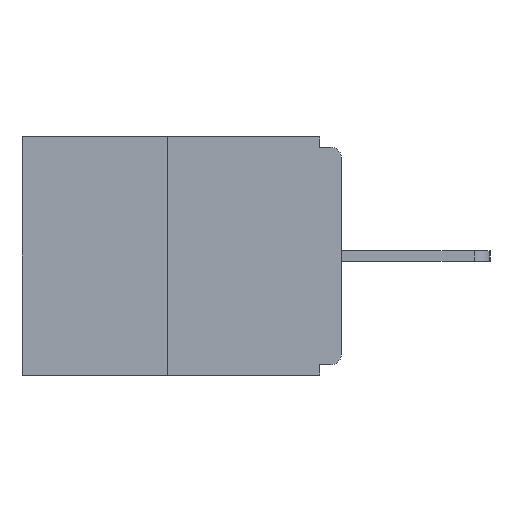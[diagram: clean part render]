
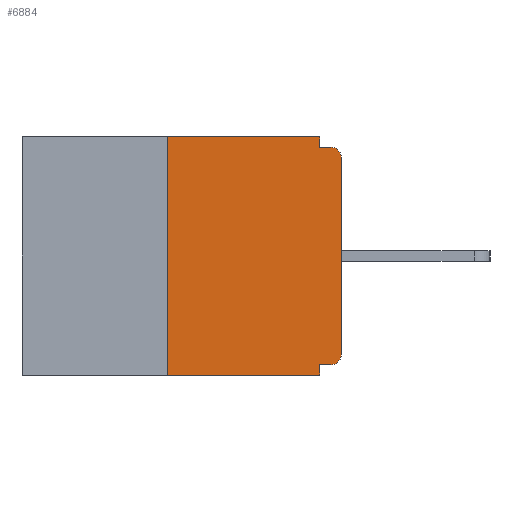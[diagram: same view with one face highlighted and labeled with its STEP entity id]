
A CAD part, left-side view. The second image highlights one B-rep face of the part: STEP entity #6884.
In plain terms, the highlighted planar face has unit normal (-1, 0, 0).
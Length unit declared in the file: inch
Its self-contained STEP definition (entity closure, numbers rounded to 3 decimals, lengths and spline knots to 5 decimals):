
#340 = CARTESIAN_POINT ( 'NONE',  ( 0., 0.031, 0. ) ) ;
#347 = DIRECTION ( 'NONE',  ( 0., 0., 1. ) ) ;
#388 = CARTESIAN_POINT ( 'NONE',  ( 0., 0.031, -0.343 ) ) ;
#733 = CARTESIAN_POINT ( 'NONE',  ( 0., 0.015, -0.313 ) ) ;
#848 = DIRECTION ( 'NONE',  ( 1., 0., 0. ) ) ;
#870 = AXIS2_PLACEMENT_3D ( 'NONE', #733, #18341, #8312 ) ;
#927 = VECTOR ( 'NONE', #15662, 39.37008 ) ;
#994 = CARTESIAN_POINT ( 'NONE',  ( 0., 0.031, 0. ) ) ;
#1183 = EDGE_CURVE ( 'NONE', #24235, #23084, #2751, .T. ) ;
#1205 = EDGE_CURVE ( 'NONE', #11519, #16282, #13908, .T. ) ;
#1241 = LINE ( 'NONE', #2749, #23325 ) ;
#1253 = CARTESIAN_POINT ( 'NONE',  ( 0., 0.031, -0.343 ) ) ;
#1765 = LINE ( 'NONE', #5658, #927 ) ;
#1881 = VERTEX_POINT ( 'NONE', #23646 ) ;
#2054 = LINE ( 'NONE', #388, #7546 ) ;
#2749 = CARTESIAN_POINT ( 'NONE',  ( 0., 0., -0.328 ) ) ;
#2751 = LINE ( 'NONE', #994, #20434 ) ;
#3595 = ORIENTED_EDGE ( 'NONE', *, *, #22627, .T. ) ;
#3606 = ORIENTED_EDGE ( 'NONE', *, *, #17704, .F. ) ;
#4128 = VECTOR ( 'NONE', #10276, 39.37008 ) ;
#4635 = LINE ( 'NONE', #17953, #11554 ) ;
#5385 = DIRECTION ( 'NONE',  ( 0., -1., 0. ) ) ;
#5658 = CARTESIAN_POINT ( 'NONE',  ( 0., 0., 0. ) ) ;
#5837 = ORIENTED_EDGE ( 'NONE', *, *, #10570, .F. ) ;
#6764 = AXIS2_PLACEMENT_3D ( 'NONE', #18196, #848, #8554 ) ;
#6884 = ADVANCED_FACE ( 'NONE', ( #14138 ), #20104, .F. ) ;
#7546 = VECTOR ( 'NONE', #21428, 39.37008 ) ;
#7661 = VERTEX_POINT ( 'NONE', #8721 ) ;
#8311 = DIRECTION ( 'NONE',  ( 0., -1., 0. ) ) ;
#8312 = DIRECTION ( 'NONE',  ( 0., 0., -1. ) ) ;
#8554 = DIRECTION ( 'NONE',  ( 0., 0., -1. ) ) ;
#8721 = CARTESIAN_POINT ( 'NONE',  ( 0., 0.015, -0.015 ) ) ;
#8810 = CARTESIAN_POINT ( 'NONE',  ( 0., 0., -0.015 ) ) ;
#9160 = VERTEX_POINT ( 'NONE', #12867 ) ;
#9673 = DIRECTION ( 'NONE',  ( 0., 0., -1. ) ) ;
#9779 = EDGE_CURVE ( 'NONE', #16980, #24235, #14578, .T. ) ;
#10276 = DIRECTION ( 'NONE',  ( 0., -1., 0. ) ) ;
#10570 = EDGE_CURVE ( 'NONE', #11519, #16980, #4635, .T. ) ;
#10665 = EDGE_CURVE ( 'NONE', #23084, #7661, #20607, .T. ) ;
#11519 = VERTEX_POINT ( 'NONE', #22918 ) ;
#11554 = VECTOR ( 'NONE', #347, 39.37008 ) ;
#11784 = CIRCLE ( 'NONE', #870, 0.015 ) ;
#12117 = CIRCLE ( 'NONE', #16175, 0.015 ) ;
#12122 = CARTESIAN_POINT ( 'NONE',  ( 0., 0.46, -0.343 ) ) ;
#12736 = VECTOR ( 'NONE', #8311, 39.37008 ) ;
#12858 = ORIENTED_EDGE ( 'NONE', *, *, #1183, .F. ) ;
#12867 = CARTESIAN_POINT ( 'NONE',  ( 0., 0.015, -0.328 ) ) ;
#13166 = EDGE_CURVE ( 'NONE', #1881, #23046, #1765, .T. ) ;
#13268 = VERTEX_POINT ( 'NONE', #13645 ) ;
#13645 = CARTESIAN_POINT ( 'NONE',  ( 0., 0.031, -0.328 ) ) ;
#13853 = CARTESIAN_POINT ( 'NONE',  ( 0., 0.25, 0. ) ) ;
#13908 = LINE ( 'NONE', #12122, #12736 ) ;
#14138 = FACE_OUTER_BOUND ( 'NONE', #19520, .T. ) ;
#14265 = VECTOR ( 'NONE', #5385, 39.37008 ) ;
#14578 = LINE ( 'NONE', #22322, #4128 ) ;
#15534 = ORIENTED_EDGE ( 'NONE', *, *, #9779, .F. ) ;
#15662 = DIRECTION ( 'NONE',  ( 0., 0., 1. ) ) ;
#16175 = AXIS2_PLACEMENT_3D ( 'NONE', #17036, #21460, #9673 ) ;
#16282 = VERTEX_POINT ( 'NONE', #1253 ) ;
#16980 = VERTEX_POINT ( 'NONE', #13853 ) ;
#17036 = CARTESIAN_POINT ( 'NONE',  ( 0., 0.015, -0.03 ) ) ;
#17704 = EDGE_CURVE ( 'NONE', #9160, #13268, #1241, .T. ) ;
#17953 = CARTESIAN_POINT ( 'NONE',  ( 0., 0.25, 0. ) ) ;
#18196 = CARTESIAN_POINT ( 'NONE',  ( 0., 0.46, 0. ) ) ;
#18341 = DIRECTION ( 'NONE',  ( -1., 0., 0. ) ) ;
#18813 = EDGE_CURVE ( 'NONE', #13268, #16282, #2054, .T. ) ;
#19520 = EDGE_LOOP ( 'NONE', ( #15534, #5837, #24483, #22707, #3606, #3595, #19781, #23598, #20793, #12858 ) ) ;
#19781 = ORIENTED_EDGE ( 'NONE', *, *, #13166, .T. ) ;
#19864 = DIRECTION ( 'NONE',  ( 0., 0., -1. ) ) ;
#20104 = PLANE ( 'NONE',  #6764 ) ;
#20434 = VECTOR ( 'NONE', #19864, 39.37008 ) ;
#20607 = LINE ( 'NONE', #8810, #14265 ) ;
#20793 = ORIENTED_EDGE ( 'NONE', *, *, #10665, .F. ) ;
#21428 = DIRECTION ( 'NONE',  ( 0., 0., -1. ) ) ;
#21460 = DIRECTION ( 'NONE',  ( -1., 0., 0. ) ) ;
#22322 = CARTESIAN_POINT ( 'NONE',  ( 0., 0.46, 0. ) ) ;
#22627 = EDGE_CURVE ( 'NONE', #9160, #1881, #11784, .T. ) ;
#22707 = ORIENTED_EDGE ( 'NONE', *, *, #18813, .F. ) ;
#22918 = CARTESIAN_POINT ( 'NONE',  ( 0., 0.25, -0.343 ) ) ;
#23046 = VERTEX_POINT ( 'NONE', #24020 ) ;
#23084 = VERTEX_POINT ( 'NONE', #23511 ) ;
#23325 = VECTOR ( 'NONE', #24425, 39.37008 ) ;
#23333 = EDGE_CURVE ( 'NONE', #23046, #7661, #12117, .T. ) ;
#23511 = CARTESIAN_POINT ( 'NONE',  ( 0., 0.031, -0.015 ) ) ;
#23598 = ORIENTED_EDGE ( 'NONE', *, *, #23333, .T. ) ;
#23646 = CARTESIAN_POINT ( 'NONE',  ( 0., 0., -0.313 ) ) ;
#24020 = CARTESIAN_POINT ( 'NONE',  ( 0., 0., -0.03 ) ) ;
#24235 = VERTEX_POINT ( 'NONE', #340 ) ;
#24425 = DIRECTION ( 'NONE',  ( 0., 1., 0. ) ) ;
#24483 = ORIENTED_EDGE ( 'NONE', *, *, #1205, .T. ) ;
